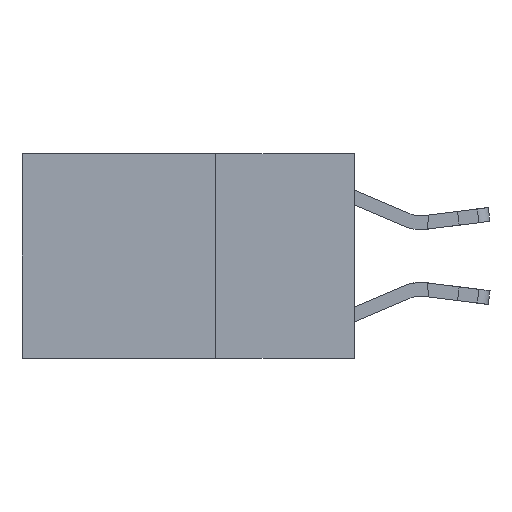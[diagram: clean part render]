
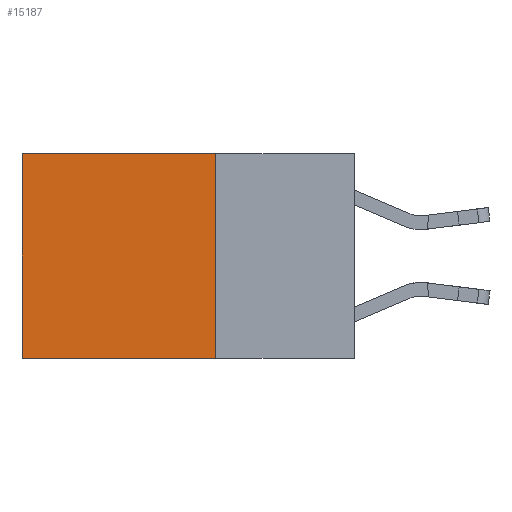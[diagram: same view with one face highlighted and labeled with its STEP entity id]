
A CAD part, left-side view. The second image highlights one B-rep face of the part: STEP entity #15187.
In plain terms, the highlighted planar face has unit normal (-1, 0, 0).
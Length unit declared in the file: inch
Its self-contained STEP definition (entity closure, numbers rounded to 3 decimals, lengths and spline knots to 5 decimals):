
#1396 = FACE_OUTER_BOUND ( 'NONE', #15779, .T. ) ;
#1891 = CARTESIAN_POINT ( 'NONE',  ( 0.2625, 0.25, -0.37 ) ) ;
#2037 = CARTESIAN_POINT ( 'NONE',  ( 0.2625, 0.25, 0. ) ) ;
#2718 = VERTEX_POINT ( 'NONE', #1891 ) ;
#4995 = ORIENTED_EDGE ( 'NONE', *, *, #6460, .T. ) ;
#5357 = CARTESIAN_POINT ( 'NONE',  ( 0.2625, 0.25, 0. ) ) ;
#6350 = LINE ( 'NONE', #7926, #16982 ) ;
#6460 = EDGE_CURVE ( 'NONE', #7944, #16823, #6350, .T. ) ;
#6575 = DIRECTION ( 'NONE',  ( 0., 0., -1. ) ) ;
#6756 = VECTOR ( 'NONE', #8564, 39.37008 ) ;
#7084 = CARTESIAN_POINT ( 'NONE',  ( 0.2625, 0.6, 0. ) ) ;
#7138 = PLANE ( 'NONE',  #11163 ) ;
#7247 = LINE ( 'NONE', #11302, #12040 ) ;
#7926 = CARTESIAN_POINT ( 'NONE',  ( 0.2625, 0.6, 0. ) ) ;
#7944 = VERTEX_POINT ( 'NONE', #7084 ) ;
#8564 = DIRECTION ( 'NONE',  ( 0., 1., 0. ) ) ;
#9613 = ORIENTED_EDGE ( 'NONE', *, *, #11618, .F. ) ;
#9838 = DIRECTION ( 'NONE',  ( 1., 0., 0. ) ) ;
#11163 = AXIS2_PLACEMENT_3D ( 'NONE', #12859, #9838, #11468 ) ;
#11302 = CARTESIAN_POINT ( 'NONE',  ( 0.2625, 0.25, -0.37 ) ) ;
#11468 = DIRECTION ( 'NONE',  ( 0., 0., -1. ) ) ;
#11618 = EDGE_CURVE ( 'NONE', #17440, #2718, #16747, .T. ) ;
#12004 = VECTOR ( 'NONE', #6575, 39.37008 ) ;
#12040 = VECTOR ( 'NONE', #17054, 39.37008 ) ;
#12074 = DIRECTION ( 'NONE',  ( 0., 0., -1. ) ) ;
#12859 = CARTESIAN_POINT ( 'NONE',  ( 0.2625, 0.25, 0. ) ) ;
#13015 = ORIENTED_EDGE ( 'NONE', *, *, #14730, .F. ) ;
#14066 = EDGE_CURVE ( 'NONE', #17440, #7944, #17515, .T. ) ;
#14730 = EDGE_CURVE ( 'NONE', #2718, #16823, #7247, .T. ) ;
#15125 = ORIENTED_EDGE ( 'NONE', *, *, #14066, .T. ) ;
#15187 = ADVANCED_FACE ( 'NONE', ( #1396 ), #7138, .F. ) ;
#15779 = EDGE_LOOP ( 'NONE', ( #4995, #13015, #9613, #15125 ) ) ;
#15845 = CARTESIAN_POINT ( 'NONE',  ( 0.2625, 0.6, -0.37 ) ) ;
#16747 = LINE ( 'NONE', #5357, #12004 ) ;
#16823 = VERTEX_POINT ( 'NONE', #15845 ) ;
#16982 = VECTOR ( 'NONE', #12074, 39.37008 ) ;
#17054 = DIRECTION ( 'NONE',  ( 0., 1., 0. ) ) ;
#17327 = CARTESIAN_POINT ( 'NONE',  ( 0.2625, 0.25, 0. ) ) ;
#17440 = VERTEX_POINT ( 'NONE', #2037 ) ;
#17515 = LINE ( 'NONE', #17327, #6756 ) ;
